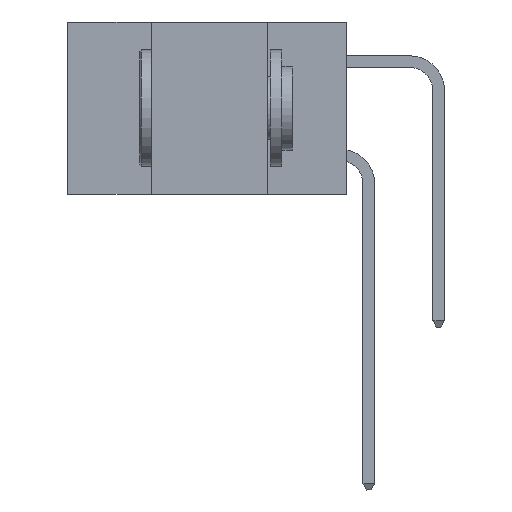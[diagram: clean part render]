
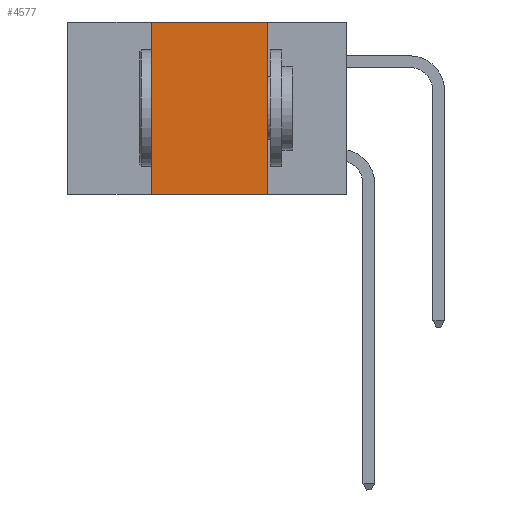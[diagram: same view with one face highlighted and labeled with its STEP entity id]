
A CAD part, left-side view. The second image highlights one B-rep face of the part: STEP entity #4577.
In plain terms, the highlighted planar face has unit normal (-1, 0, 0).
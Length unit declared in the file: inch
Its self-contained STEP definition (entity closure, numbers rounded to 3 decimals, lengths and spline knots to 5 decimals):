
#22 = CARTESIAN_POINT ( 'NONE',  ( 0., 0.17, 0. ) ) ;
#850 = ORIENTED_EDGE ( 'NONE', *, *, #5390, .F. ) ;
#1006 = DIRECTION ( 'NONE',  ( 1., 0., 0. ) ) ;
#1472 = EDGE_CURVE ( 'NONE', #2063, #11327, #2103, .T. ) ;
#2063 = VERTEX_POINT ( 'NONE', #5394 ) ;
#2103 = LINE ( 'NONE', #6978, #13135 ) ;
#2472 = EDGE_CURVE ( 'NONE', #12368, #14475, #2722, .T. ) ;
#2590 = LINE ( 'NONE', #7020, #8461 ) ;
#2722 = LINE ( 'NONE', #7728, #10746 ) ;
#2796 = CARTESIAN_POINT ( 'NONE',  ( 0., 0.42, -0.37 ) ) ;
#3613 = CARTESIAN_POINT ( 'NONE',  ( 0., 0.17, -0.37 ) ) ;
#4373 = ORIENTED_EDGE ( 'NONE', *, *, #1472, .F. ) ;
#4404 = DIRECTION ( 'NONE',  ( 0., 0., 1. ) ) ;
#4577 = ADVANCED_FACE ( 'NONE', ( #12622 ), #17482, .F. ) ;
#5190 = LINE ( 'NONE', #16396, #12295 ) ;
#5390 = EDGE_CURVE ( 'NONE', #11327, #14475, #5190, .T. ) ;
#5394 = CARTESIAN_POINT ( 'NONE',  ( 0., 0.42, 0. ) ) ;
#6250 = EDGE_LOOP ( 'NONE', ( #850, #4373, #15899, #15878 ) ) ;
#6978 = CARTESIAN_POINT ( 'NONE',  ( 0., 0.6, 0. ) ) ;
#7020 = CARTESIAN_POINT ( 'NONE',  ( 0., 0.42, 0. ) ) ;
#7728 = CARTESIAN_POINT ( 'NONE',  ( 0., 0.6, -0.37 ) ) ;
#8350 = DIRECTION ( 'NONE',  ( 0., -1., 0. ) ) ;
#8461 = VECTOR ( 'NONE', #4404, 39.37008 ) ;
#9235 = DIRECTION ( 'NONE',  ( 0., 0., -1. ) ) ;
#9574 = DIRECTION ( 'NONE',  ( 0., 0., -1. ) ) ;
#9624 = AXIS2_PLACEMENT_3D ( 'NONE', #14613, #1006, #9235 ) ;
#10746 = VECTOR ( 'NONE', #13245, 39.37008 ) ;
#11327 = VERTEX_POINT ( 'NONE', #22 ) ;
#12295 = VECTOR ( 'NONE', #9574, 39.37008 ) ;
#12368 = VERTEX_POINT ( 'NONE', #2796 ) ;
#12622 = FACE_OUTER_BOUND ( 'NONE', #6250, .T. ) ;
#13135 = VECTOR ( 'NONE', #8350, 39.37008 ) ;
#13245 = DIRECTION ( 'NONE',  ( 0., -1., 0. ) ) ;
#14475 = VERTEX_POINT ( 'NONE', #3613 ) ;
#14613 = CARTESIAN_POINT ( 'NONE',  ( 0., 0.6, 0. ) ) ;
#15878 = ORIENTED_EDGE ( 'NONE', *, *, #2472, .T. ) ;
#15899 = ORIENTED_EDGE ( 'NONE', *, *, #16667, .F. ) ;
#16396 = CARTESIAN_POINT ( 'NONE',  ( 0., 0.17, 0. ) ) ;
#16667 = EDGE_CURVE ( 'NONE', #12368, #2063, #2590, .T. ) ;
#17482 = PLANE ( 'NONE',  #9624 ) ;
